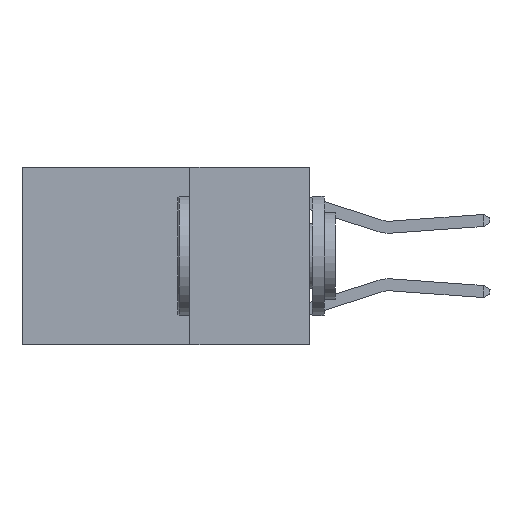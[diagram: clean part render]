
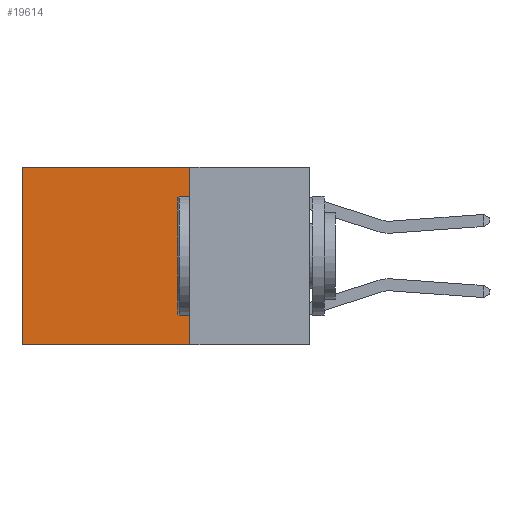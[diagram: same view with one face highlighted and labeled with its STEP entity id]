
A CAD part, left-side view. The second image highlights one B-rep face of the part: STEP entity #19614.
In plain terms, the highlighted planar face has unit normal (-1, 0, 0).
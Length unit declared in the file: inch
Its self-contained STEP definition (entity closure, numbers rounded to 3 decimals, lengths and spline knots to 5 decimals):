
#343 = ORIENTED_EDGE ( 'NONE', *, *, #3212, .F. ) ;
#2227 = DIRECTION ( 'NONE',  ( 0., 0., -1. ) ) ;
#3050 = CARTESIAN_POINT ( 'NONE',  ( 0.2625, 0.25, 0. ) ) ;
#3156 = DIRECTION ( 'NONE',  ( 0., 0., -1. ) ) ;
#3212 = EDGE_CURVE ( 'NONE', #16702, #13024, #8441, .T. ) ;
#3217 = EDGE_CURVE ( 'NONE', #5459, #10080, #3259, .T. ) ;
#3259 = LINE ( 'NONE', #17716, #6722 ) ;
#4107 = CARTESIAN_POINT ( 'NONE',  ( 0.2625, 0.6, 0. ) ) ;
#5459 = VERTEX_POINT ( 'NONE', #4107 ) ;
#5909 = DIRECTION ( 'NONE',  ( 0., 1., 0. ) ) ;
#6244 = VECTOR ( 'NONE', #21330, 39.37008 ) ;
#6340 = EDGE_CURVE ( 'NONE', #13024, #10080, #12108, .T. ) ;
#6722 = VECTOR ( 'NONE', #19927, 39.37008 ) ;
#7173 = CARTESIAN_POINT ( 'NONE',  ( 0.2625, 0.25, -0.37 ) ) ;
#7408 = CARTESIAN_POINT ( 'NONE',  ( 0.2625, 0.25, -0.37 ) ) ;
#8441 = LINE ( 'NONE', #12694, #9122 ) ;
#8560 = AXIS2_PLACEMENT_3D ( 'NONE', #3050, #9626, #3156 ) ;
#8809 = ORIENTED_EDGE ( 'NONE', *, *, #6340, .F. ) ;
#9122 = VECTOR ( 'NONE', #2227, 39.37008 ) ;
#9626 = DIRECTION ( 'NONE',  ( 1., 0., 0. ) ) ;
#9857 = ORIENTED_EDGE ( 'NONE', *, *, #13945, .T. ) ;
#9863 = CARTESIAN_POINT ( 'NONE',  ( 0.2625, 0.6, -0.37 ) ) ;
#10080 = VERTEX_POINT ( 'NONE', #9863 ) ;
#12108 = LINE ( 'NONE', #7408, #6244 ) ;
#12694 = CARTESIAN_POINT ( 'NONE',  ( 0.2625, 0.25, 0. ) ) ;
#12746 = CARTESIAN_POINT ( 'NONE',  ( 0.2625, 0.25, 0. ) ) ;
#12819 = CARTESIAN_POINT ( 'NONE',  ( 0.2625, 0.25, 0. ) ) ;
#13024 = VERTEX_POINT ( 'NONE', #7173 ) ;
#13945 = EDGE_CURVE ( 'NONE', #16702, #5459, #22893, .T. ) ;
#14290 = FACE_OUTER_BOUND ( 'NONE', #14493, .T. ) ;
#14493 = EDGE_LOOP ( 'NONE', ( #28228, #8809, #343, #9857 ) ) ;
#16702 = VERTEX_POINT ( 'NONE', #12819 ) ;
#17716 = CARTESIAN_POINT ( 'NONE',  ( 0.2625, 0.6, 0. ) ) ;
#18384 = VECTOR ( 'NONE', #5909, 39.37008 ) ;
#19614 = ADVANCED_FACE ( 'NONE', ( #14290 ), #23010, .F. ) ;
#19927 = DIRECTION ( 'NONE',  ( 0., 0., -1. ) ) ;
#21330 = DIRECTION ( 'NONE',  ( 0., 1., 0. ) ) ;
#22893 = LINE ( 'NONE', #12746, #18384 ) ;
#23010 = PLANE ( 'NONE',  #8560 ) ;
#28228 = ORIENTED_EDGE ( 'NONE', *, *, #3217, .T. ) ;
